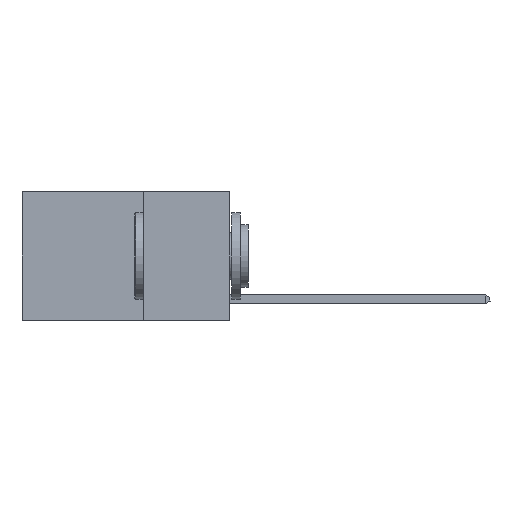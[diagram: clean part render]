
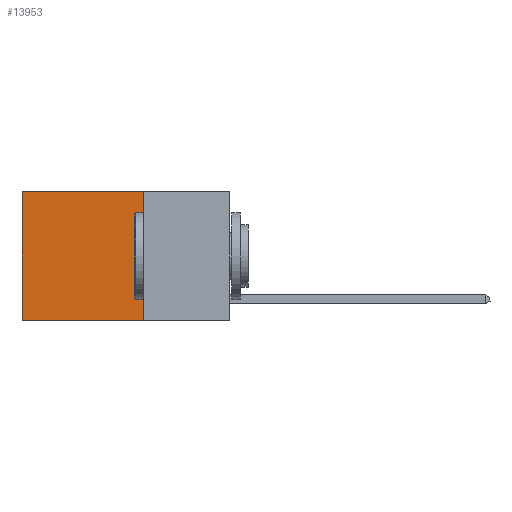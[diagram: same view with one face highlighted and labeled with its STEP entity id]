
A CAD part, left-side view. The second image highlights one B-rep face of the part: STEP entity #13953.
In plain terms, the highlighted planar face has unit normal (-1, 0, 0).
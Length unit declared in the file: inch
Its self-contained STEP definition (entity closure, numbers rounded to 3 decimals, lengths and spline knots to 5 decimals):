
#185 = EDGE_CURVE ( 'NONE', #7051, #5643, #13617, .T. ) ;
#749 = VECTOR ( 'NONE', #5909, 39.37008 ) ;
#1016 = DIRECTION ( 'NONE',  ( 0., 0., -1. ) ) ;
#1024 = CARTESIAN_POINT ( 'NONE',  ( 0.2625, 0.25, -0.37 ) ) ;
#1123 = CARTESIAN_POINT ( 'NONE',  ( 0.2625, 0.25, -0.37 ) ) ;
#1129 = VECTOR ( 'NONE', #4325, 39.37008 ) ;
#1172 = CARTESIAN_POINT ( 'NONE',  ( 0.2625, 0.25, 0. ) ) ;
#1946 = CARTESIAN_POINT ( 'NONE',  ( 0.2625, 0.6, 0. ) ) ;
#2809 = EDGE_CURVE ( 'NONE', #11028, #5660, #15030, .T. ) ;
#2917 = LINE ( 'NONE', #7849, #8773 ) ;
#4084 = EDGE_CURVE ( 'NONE', #7051, #11028, #2917, .T. ) ;
#4325 = DIRECTION ( 'NONE',  ( 0., 0., -1. ) ) ;
#4648 = CARTESIAN_POINT ( 'NONE',  ( 0.2625, 0.6, -0.37 ) ) ;
#5391 = CARTESIAN_POINT ( 'NONE',  ( 0.2625, 0.25, 0. ) ) ;
#5415 = CARTESIAN_POINT ( 'NONE',  ( 0.2625, 0.25, 0. ) ) ;
#5643 = VERTEX_POINT ( 'NONE', #1024 ) ;
#5660 = VERTEX_POINT ( 'NONE', #4648 ) ;
#5909 = DIRECTION ( 'NONE',  ( 0., 1., 0. ) ) ;
#6110 = FACE_OUTER_BOUND ( 'NONE', #12877, .T. ) ;
#6411 = EDGE_CURVE ( 'NONE', #5643, #5660, #14203, .T. ) ;
#6523 = DIRECTION ( 'NONE',  ( 0., 1., 0. ) ) ;
#7051 = VERTEX_POINT ( 'NONE', #5415 ) ;
#7659 = DIRECTION ( 'NONE',  ( 0., 0., -1. ) ) ;
#7849 = CARTESIAN_POINT ( 'NONE',  ( 0.2625, 0.25, 0. ) ) ;
#8773 = VECTOR ( 'NONE', #6523, 39.37008 ) ;
#9349 = ORIENTED_EDGE ( 'NONE', *, *, #4084, .T. ) ;
#10386 = VECTOR ( 'NONE', #7659, 39.37008 ) ;
#10401 = AXIS2_PLACEMENT_3D ( 'NONE', #1172, #15442, #1016 ) ;
#10657 = ORIENTED_EDGE ( 'NONE', *, *, #2809, .T. ) ;
#11028 = VERTEX_POINT ( 'NONE', #15344 ) ;
#11761 = PLANE ( 'NONE',  #10401 ) ;
#12877 = EDGE_LOOP ( 'NONE', ( #10657, #14206, #13731, #9349 ) ) ;
#13617 = LINE ( 'NONE', #5391, #10386 ) ;
#13731 = ORIENTED_EDGE ( 'NONE', *, *, #185, .F. ) ;
#13953 = ADVANCED_FACE ( 'NONE', ( #6110 ), #11761, .F. ) ;
#14203 = LINE ( 'NONE', #1123, #749 ) ;
#14206 = ORIENTED_EDGE ( 'NONE', *, *, #6411, .F. ) ;
#15030 = LINE ( 'NONE', #1946, #1129 ) ;
#15344 = CARTESIAN_POINT ( 'NONE',  ( 0.2625, 0.6, 0. ) ) ;
#15442 = DIRECTION ( 'NONE',  ( 1., 0., 0. ) ) ;
